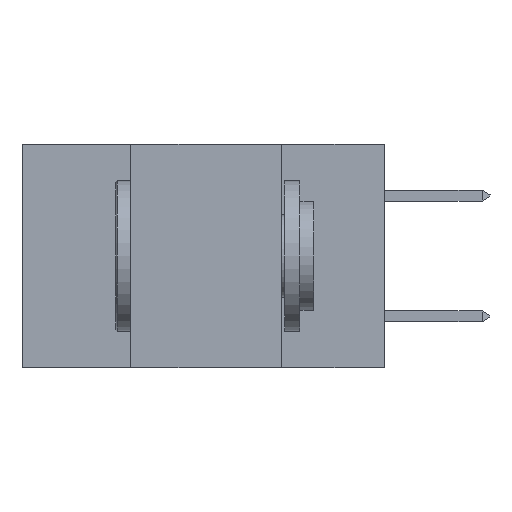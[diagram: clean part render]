
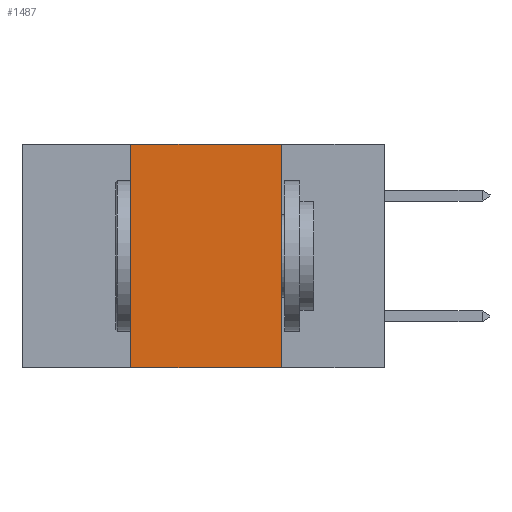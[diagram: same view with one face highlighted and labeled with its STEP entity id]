
A CAD part, left-side view. The second image highlights one B-rep face of the part: STEP entity #1487.
In plain terms, the highlighted planar face has unit normal (-1, 0, 0).
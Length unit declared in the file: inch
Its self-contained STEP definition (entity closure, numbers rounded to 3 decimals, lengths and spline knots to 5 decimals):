
#598 = AXIS2_PLACEMENT_3D ( 'NONE', #10264, #7619, #16848 ) ;
#753 = PLANE ( 'NONE',  #598 ) ;
#879 = VECTOR ( 'NONE', #8292, 39.37008 ) ;
#1434 = DIRECTION ( 'NONE',  ( 0., 0., -1. ) ) ;
#1487 = ADVANCED_FACE ( 'NONE', ( #2349 ), #753, .F. ) ;
#1907 = EDGE_LOOP ( 'NONE', ( #2007, #16769, #2814, #4982 ) ) ;
#2007 = ORIENTED_EDGE ( 'NONE', *, *, #3489, .F. ) ;
#2349 = FACE_OUTER_BOUND ( 'NONE', #1907, .T. ) ;
#2814 = ORIENTED_EDGE ( 'NONE', *, *, #15997, .F. ) ;
#3489 = EDGE_CURVE ( 'NONE', #11180, #12368, #16462, .T. ) ;
#3835 = CARTESIAN_POINT ( 'NONE',  ( 0., 0.42, -0.37 ) ) ;
#4222 = CARTESIAN_POINT ( 'NONE',  ( 0., 0.17, 0. ) ) ;
#4605 = CARTESIAN_POINT ( 'NONE',  ( 0., 0.17, -0.37 ) ) ;
#4982 = ORIENTED_EDGE ( 'NONE', *, *, #11644, .T. ) ;
#4990 = VERTEX_POINT ( 'NONE', #3835 ) ;
#6075 = EDGE_CURVE ( 'NONE', #11490, #11180, #9369, .T. ) ;
#6305 = CARTESIAN_POINT ( 'NONE',  ( 0., 0.42, 0. ) ) ;
#6333 = DIRECTION ( 'NONE',  ( 0., -1., 0. ) ) ;
#7062 = CARTESIAN_POINT ( 'NONE',  ( 0., 0.17, 0. ) ) ;
#7619 = DIRECTION ( 'NONE',  ( 1., 0., 0. ) ) ;
#7807 = VECTOR ( 'NONE', #6333, 39.37008 ) ;
#8292 = DIRECTION ( 'NONE',  ( 0., -1., 0. ) ) ;
#8367 = CARTESIAN_POINT ( 'NONE',  ( 0., 0.6, 0. ) ) ;
#8986 = CARTESIAN_POINT ( 'NONE',  ( 0., 0.6, -0.37 ) ) ;
#9369 = LINE ( 'NONE', #8367, #879 ) ;
#10264 = CARTESIAN_POINT ( 'NONE',  ( 0., 0.6, 0. ) ) ;
#11180 = VERTEX_POINT ( 'NONE', #7062 ) ;
#11490 = VERTEX_POINT ( 'NONE', #12476 ) ;
#11644 = EDGE_CURVE ( 'NONE', #4990, #12368, #14159, .T. ) ;
#11917 = DIRECTION ( 'NONE',  ( 0., 0., 1. ) ) ;
#12368 = VERTEX_POINT ( 'NONE', #4605 ) ;
#12476 = CARTESIAN_POINT ( 'NONE',  ( 0., 0.42, 0. ) ) ;
#14159 = LINE ( 'NONE', #8986, #7807 ) ;
#14338 = VECTOR ( 'NONE', #1434, 39.37008 ) ;
#15997 = EDGE_CURVE ( 'NONE', #4990, #11490, #16962, .T. ) ;
#16462 = LINE ( 'NONE', #4222, #14338 ) ;
#16769 = ORIENTED_EDGE ( 'NONE', *, *, #6075, .F. ) ;
#16848 = DIRECTION ( 'NONE',  ( 0., 0., -1. ) ) ;
#16962 = LINE ( 'NONE', #6305, #17394 ) ;
#17394 = VECTOR ( 'NONE', #11917, 39.37008 ) ;
